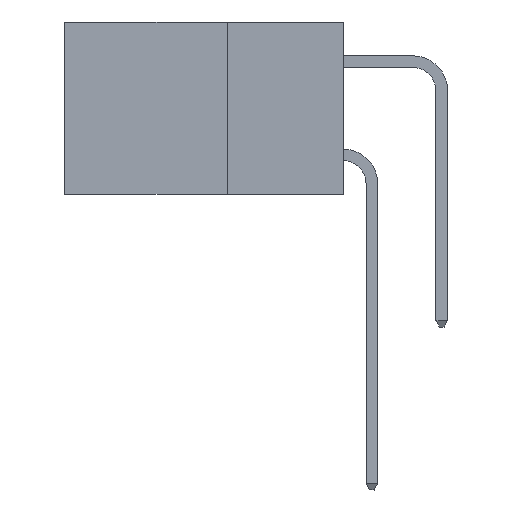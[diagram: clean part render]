
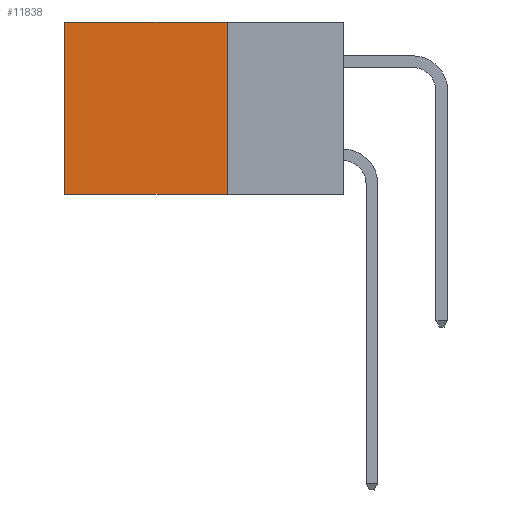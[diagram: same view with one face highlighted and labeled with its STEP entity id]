
A CAD part, left-side view. The second image highlights one B-rep face of the part: STEP entity #11838.
In plain terms, the highlighted planar face has unit normal (-1, 0, 0).
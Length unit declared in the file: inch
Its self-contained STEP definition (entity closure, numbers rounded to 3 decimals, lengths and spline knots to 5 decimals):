
#431 = CARTESIAN_POINT ( 'NONE',  ( 0.2615, 0.25, -0.37 ) ) ;
#925 = CARTESIAN_POINT ( 'NONE',  ( 0.2615, 0.25, -0.37 ) ) ;
#1381 = DIRECTION ( 'NONE',  ( 0., 1., 0. ) ) ;
#1642 = LINE ( 'NONE', #19482, #25355 ) ;
#1969 = CARTESIAN_POINT ( 'NONE',  ( 0.2615, 0.25, -0.37 ) ) ;
#2398 = ORIENTED_EDGE ( 'NONE', *, *, #10077, .F. ) ;
#4474 = ORIENTED_EDGE ( 'NONE', *, *, #15383, .T. ) ;
#4601 = FACE_OUTER_BOUND ( 'NONE', #20196, .T. ) ;
#6429 = PLANE ( 'NONE',  #21230 ) ;
#7389 = EDGE_CURVE ( 'NONE', #24760, #23542, #14116, .T. ) ;
#9868 = EDGE_CURVE ( 'NONE', #24760, #12368, #1642, .T. ) ;
#9963 = DIRECTION ( 'NONE',  ( 0., 0., -1. ) ) ;
#10077 = EDGE_CURVE ( 'NONE', #23542, #17073, #11377, .T. ) ;
#10471 = LINE ( 'NONE', #22333, #18265 ) ;
#11377 = LINE ( 'NONE', #22995, #18261 ) ;
#11739 = CARTESIAN_POINT ( 'NONE',  ( 0.2615, 0.6, -0.37 ) ) ;
#11838 = ADVANCED_FACE ( 'NONE', ( #4601 ), #6429, .F. ) ;
#12024 = DIRECTION ( 'NONE',  ( 0., 0., -1. ) ) ;
#12368 = VERTEX_POINT ( 'NONE', #23288 ) ;
#12924 = DIRECTION ( 'NONE',  ( 0., 0., -1. ) ) ;
#14116 = LINE ( 'NONE', #431, #22737 ) ;
#14673 = CARTESIAN_POINT ( 'NONE',  ( 0.2615, 0.25, 0. ) ) ;
#15383 = EDGE_CURVE ( 'NONE', #12368, #17073, #10471, .T. ) ;
#17073 = VERTEX_POINT ( 'NONE', #11739 ) ;
#18261 = VECTOR ( 'NONE', #19310, 39.37008 ) ;
#18265 = VECTOR ( 'NONE', #12024, 39.37008 ) ;
#19310 = DIRECTION ( 'NONE',  ( 0., 1., 0. ) ) ;
#19482 = CARTESIAN_POINT ( 'NONE',  ( 0.2615, 0.25, 0. ) ) ;
#20196 = EDGE_LOOP ( 'NONE', ( #4474, #2398, #23895, #25416 ) ) ;
#20335 = DIRECTION ( 'NONE',  ( 1., 0., 0. ) ) ;
#21230 = AXIS2_PLACEMENT_3D ( 'NONE', #925, #20335, #12924 ) ;
#22333 = CARTESIAN_POINT ( 'NONE',  ( 0.2615, 0.6, -0.37 ) ) ;
#22737 = VECTOR ( 'NONE', #9963, 39.37008 ) ;
#22995 = CARTESIAN_POINT ( 'NONE',  ( 0.2615, 0.25, -0.37 ) ) ;
#23288 = CARTESIAN_POINT ( 'NONE',  ( 0.2615, 0.6, 0. ) ) ;
#23542 = VERTEX_POINT ( 'NONE', #1969 ) ;
#23895 = ORIENTED_EDGE ( 'NONE', *, *, #7389, .F. ) ;
#24760 = VERTEX_POINT ( 'NONE', #14673 ) ;
#25355 = VECTOR ( 'NONE', #1381, 39.37008 ) ;
#25416 = ORIENTED_EDGE ( 'NONE', *, *, #9868, .T. ) ;
